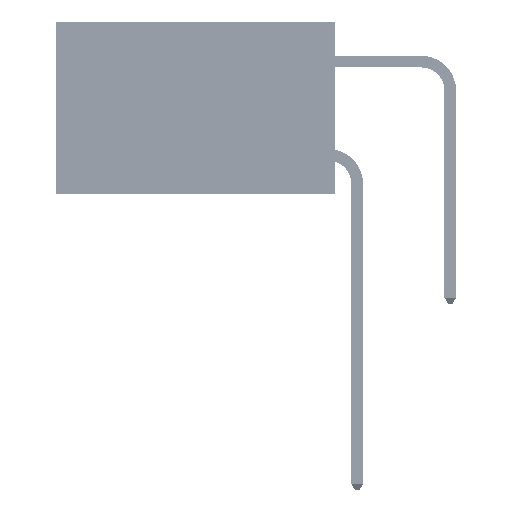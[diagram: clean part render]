
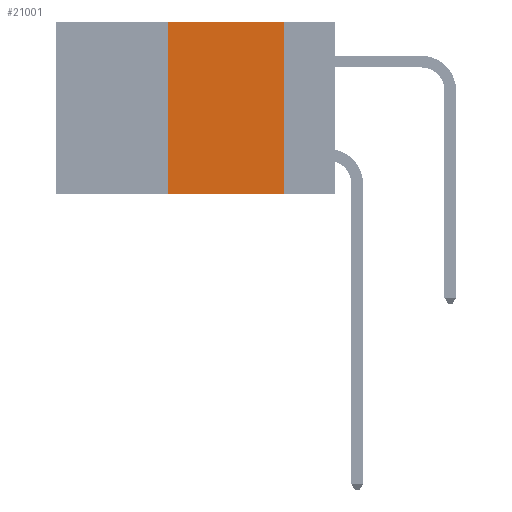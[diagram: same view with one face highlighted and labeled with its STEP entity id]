
A CAD part, left-side view. The second image highlights one B-rep face of the part: STEP entity #21001.
In plain terms, the highlighted planar face has unit normal (-1, 0, 0).
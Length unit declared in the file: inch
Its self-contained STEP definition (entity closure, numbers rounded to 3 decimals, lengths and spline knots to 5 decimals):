
#608 = VECTOR ( 'NONE', #25796, 39.37008 ) ;
#792 = DIRECTION ( 'NONE',  ( 0., 0., -1. ) ) ;
#1214 = CARTESIAN_POINT ( 'NONE',  ( 0., 0.6, -0.37 ) ) ;
#3380 = CARTESIAN_POINT ( 'NONE',  ( 0., 0.36, -0.37 ) ) ;
#6517 = CARTESIAN_POINT ( 'NONE',  ( 0., 0.6, 0. ) ) ;
#7070 = VERTEX_POINT ( 'NONE', #11262 ) ;
#11262 = CARTESIAN_POINT ( 'NONE',  ( 0., 0.11, 0. ) ) ;
#12287 = VERTEX_POINT ( 'NONE', #36097 ) ;
#15185 = VERTEX_POINT ( 'NONE', #22789 ) ;
#16809 = LINE ( 'NONE', #41196, #608 ) ;
#17502 = EDGE_CURVE ( 'NONE', #12287, #7070, #16809, .T. ) ;
#20492 = VERTEX_POINT ( 'NONE', #3380 ) ;
#20911 = ORIENTED_EDGE ( 'NONE', *, *, #27595, .F. ) ;
#21001 = ADVANCED_FACE ( 'NONE', ( #21076 ), #44860, .F. ) ;
#21076 = FACE_OUTER_BOUND ( 'NONE', #31910, .T. ) ;
#21917 = DIRECTION ( 'NONE',  ( 1., 0., 0. ) ) ;
#22789 = CARTESIAN_POINT ( 'NONE',  ( 0., 0.11, -0.37 ) ) ;
#22951 = AXIS2_PLACEMENT_3D ( 'NONE', #6517, #21917, #45022 ) ;
#23013 = VECTOR ( 'NONE', #26157, 39.37008 ) ;
#25466 = LINE ( 'NONE', #1214, #30879 ) ;
#25796 = DIRECTION ( 'NONE',  ( 0., -1., 0. ) ) ;
#26157 = DIRECTION ( 'NONE',  ( 0., 0., 1. ) ) ;
#27403 = DIRECTION ( 'NONE',  ( 0., -1., 0. ) ) ;
#27595 = EDGE_CURVE ( 'NONE', #7070, #15185, #43928, .T. ) ;
#30834 = ORIENTED_EDGE ( 'NONE', *, *, #17502, .F. ) ;
#30879 = VECTOR ( 'NONE', #27403, 39.37008 ) ;
#31491 = LINE ( 'NONE', #40909, #23013 ) ;
#31910 = EDGE_LOOP ( 'NONE', ( #20911, #30834, #37000, #36455 ) ) ;
#36097 = CARTESIAN_POINT ( 'NONE',  ( 0., 0.36, 0. ) ) ;
#36455 = ORIENTED_EDGE ( 'NONE', *, *, #49417, .T. ) ;
#37000 = ORIENTED_EDGE ( 'NONE', *, *, #43250, .F. ) ;
#40909 = CARTESIAN_POINT ( 'NONE',  ( 0., 0.36, 0. ) ) ;
#41196 = CARTESIAN_POINT ( 'NONE',  ( 0., 0.6, 0. ) ) ;
#42734 = VECTOR ( 'NONE', #792, 39.37008 ) ;
#43250 = EDGE_CURVE ( 'NONE', #20492, #12287, #31491, .T. ) ;
#43928 = LINE ( 'NONE', #46656, #42734 ) ;
#44860 = PLANE ( 'NONE',  #22951 ) ;
#45022 = DIRECTION ( 'NONE',  ( 0., 0., -1. ) ) ;
#46656 = CARTESIAN_POINT ( 'NONE',  ( 0., 0.11, 0. ) ) ;
#49417 = EDGE_CURVE ( 'NONE', #20492, #15185, #25466, .T. ) ;
